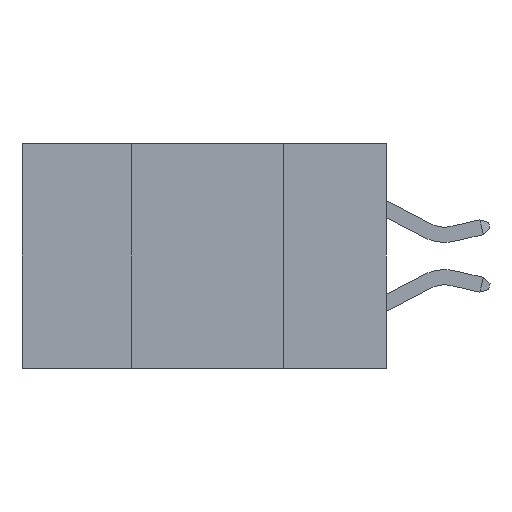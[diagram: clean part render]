
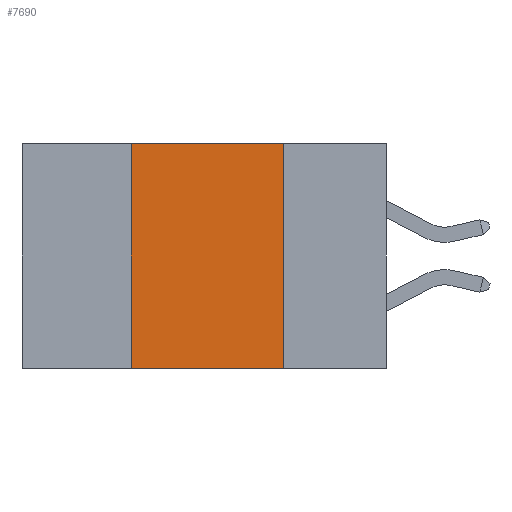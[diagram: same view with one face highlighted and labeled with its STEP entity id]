
A CAD part, left-side view. The second image highlights one B-rep face of the part: STEP entity #7690.
In plain terms, the highlighted planar face has unit normal (-1, 0, 0).
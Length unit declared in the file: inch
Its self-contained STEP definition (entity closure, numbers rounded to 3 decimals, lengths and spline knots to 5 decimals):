
#34 = DIRECTION ( 'NONE',  ( 0., -1., 0. ) ) ;
#75 = CARTESIAN_POINT ( 'NONE',  ( 0., 0.6, 0. ) ) ;
#1246 = ORIENTED_EDGE ( 'NONE', *, *, #1756, .F. ) ;
#1756 = EDGE_CURVE ( 'NONE', #4195, #15176, #7714, .T. ) ;
#1961 = DIRECTION ( 'NONE',  ( 0., 0., -1. ) ) ;
#2013 = CARTESIAN_POINT ( 'NONE',  ( 0., 0.42, -0.37 ) ) ;
#2055 = AXIS2_PLACEMENT_3D ( 'NONE', #5660, #5907, #5331 ) ;
#2065 = DIRECTION ( 'NONE',  ( 0., 0., 1. ) ) ;
#3353 = LINE ( 'NONE', #13516, #6747 ) ;
#4195 = VERTEX_POINT ( 'NONE', #7938 ) ;
#4241 = CARTESIAN_POINT ( 'NONE',  ( 0., 0.17, -0.37 ) ) ;
#4324 = FACE_OUTER_BOUND ( 'NONE', #14496, .T. ) ;
#4658 = ORIENTED_EDGE ( 'NONE', *, *, #15456, .T. ) ;
#5331 = DIRECTION ( 'NONE',  ( 0., 0., -1. ) ) ;
#5516 = PLANE ( 'NONE',  #2055 ) ;
#5660 = CARTESIAN_POINT ( 'NONE',  ( 0., 0.6, 0. ) ) ;
#5907 = DIRECTION ( 'NONE',  ( 1., 0., 0. ) ) ;
#5920 = LINE ( 'NONE', #75, #15025 ) ;
#6026 = DIRECTION ( 'NONE',  ( 0., -1., 0. ) ) ;
#6747 = VECTOR ( 'NONE', #6026, 39.37008 ) ;
#7690 = ADVANCED_FACE ( 'NONE', ( #4324 ), #5516, .F. ) ;
#7714 = LINE ( 'NONE', #2013, #13893 ) ;
#7938 = CARTESIAN_POINT ( 'NONE',  ( 0., 0.42, -0.37 ) ) ;
#8081 = CARTESIAN_POINT ( 'NONE',  ( 0., 0.42, 0. ) ) ;
#8635 = EDGE_CURVE ( 'NONE', #15176, #15195, #5920, .T. ) ;
#11023 = ORIENTED_EDGE ( 'NONE', *, *, #8635, .F. ) ;
#11925 = EDGE_CURVE ( 'NONE', #15195, #15210, #15523, .T. ) ;
#12348 = VECTOR ( 'NONE', #1961, 39.37008 ) ;
#13516 = CARTESIAN_POINT ( 'NONE',  ( 0., 0.6, -0.37 ) ) ;
#13887 = ORIENTED_EDGE ( 'NONE', *, *, #11925, .F. ) ;
#13893 = VECTOR ( 'NONE', #2065, 39.37008 ) ;
#14443 = CARTESIAN_POINT ( 'NONE',  ( 0., 0.17, -0.37 ) ) ;
#14496 = EDGE_LOOP ( 'NONE', ( #13887, #11023, #1246, #4658 ) ) ;
#15025 = VECTOR ( 'NONE', #34, 39.37008 ) ;
#15176 = VERTEX_POINT ( 'NONE', #8081 ) ;
#15195 = VERTEX_POINT ( 'NONE', #15389 ) ;
#15210 = VERTEX_POINT ( 'NONE', #4241 ) ;
#15389 = CARTESIAN_POINT ( 'NONE',  ( 0., 0.17, 0. ) ) ;
#15456 = EDGE_CURVE ( 'NONE', #4195, #15210, #3353, .T. ) ;
#15523 = LINE ( 'NONE', #14443, #12348 ) ;
